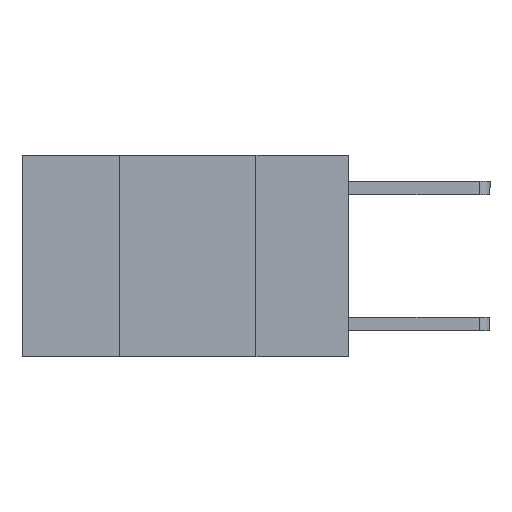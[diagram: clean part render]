
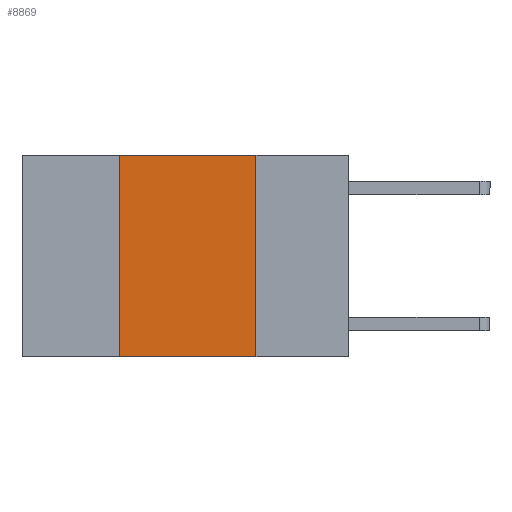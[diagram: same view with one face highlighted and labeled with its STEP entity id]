
A CAD part, left-side view. The second image highlights one B-rep face of the part: STEP entity #8869.
In plain terms, the highlighted planar face has unit normal (-1, 0, 0).
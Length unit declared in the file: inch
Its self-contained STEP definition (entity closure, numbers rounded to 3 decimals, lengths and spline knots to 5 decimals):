
#104 = EDGE_LOOP ( 'NONE', ( #6926, #2718, #4434, #5440 ) ) ;
#144 = EDGE_CURVE ( 'NONE', #7328, #1007, #1130, .T. ) ;
#227 = VECTOR ( 'NONE', #1446, 39.37008 ) ;
#294 = CARTESIAN_POINT ( 'NONE',  ( 0., 0.6, 0. ) ) ;
#667 = CARTESIAN_POINT ( 'NONE',  ( 0., 0.42, -0.37 ) ) ;
#863 = PLANE ( 'NONE',  #9332 ) ;
#979 = CARTESIAN_POINT ( 'NONE',  ( 0., 0.6, -0.37 ) ) ;
#1007 = VERTEX_POINT ( 'NONE', #3059 ) ;
#1130 = LINE ( 'NONE', #4024, #8418 ) ;
#1446 = DIRECTION ( 'NONE',  ( 0., 0., -1. ) ) ;
#1907 = LINE ( 'NONE', #4088, #3095 ) ;
#2405 = DIRECTION ( 'NONE',  ( 0., -1., 0. ) ) ;
#2706 = VECTOR ( 'NONE', #2405, 39.37008 ) ;
#2718 = ORIENTED_EDGE ( 'NONE', *, *, #5056, .F. ) ;
#3059 = CARTESIAN_POINT ( 'NONE',  ( 0., 0.42, 0. ) ) ;
#3095 = VECTOR ( 'NONE', #9239, 39.37008 ) ;
#4024 = CARTESIAN_POINT ( 'NONE',  ( 0., 0.42, 0. ) ) ;
#4088 = CARTESIAN_POINT ( 'NONE',  ( 0., 0.6, 0. ) ) ;
#4411 = VERTEX_POINT ( 'NONE', #5326 ) ;
#4434 = ORIENTED_EDGE ( 'NONE', *, *, #144, .F. ) ;
#4510 = FACE_OUTER_BOUND ( 'NONE', #104, .T. ) ;
#4603 = DIRECTION ( 'NONE',  ( 1., 0., 0. ) ) ;
#5056 = EDGE_CURVE ( 'NONE', #1007, #8896, #1907, .T. ) ;
#5326 = CARTESIAN_POINT ( 'NONE',  ( 0., 0.17, -0.37 ) ) ;
#5440 = ORIENTED_EDGE ( 'NONE', *, *, #9345, .T. ) ;
#5796 = CARTESIAN_POINT ( 'NONE',  ( 0., 0.17, 0. ) ) ;
#6628 = EDGE_CURVE ( 'NONE', #8896, #4411, #7937, .T. ) ;
#6716 = LINE ( 'NONE', #979, #2706 ) ;
#6791 = CARTESIAN_POINT ( 'NONE',  ( 0., 0.17, 0. ) ) ;
#6904 = DIRECTION ( 'NONE',  ( 0., 0., 1. ) ) ;
#6926 = ORIENTED_EDGE ( 'NONE', *, *, #6628, .F. ) ;
#7328 = VERTEX_POINT ( 'NONE', #667 ) ;
#7937 = LINE ( 'NONE', #5796, #227 ) ;
#8418 = VECTOR ( 'NONE', #6904, 39.37008 ) ;
#8757 = DIRECTION ( 'NONE',  ( 0., 0., -1. ) ) ;
#8869 = ADVANCED_FACE ( 'NONE', ( #4510 ), #863, .F. ) ;
#8896 = VERTEX_POINT ( 'NONE', #6791 ) ;
#9239 = DIRECTION ( 'NONE',  ( 0., -1., 0. ) ) ;
#9332 = AXIS2_PLACEMENT_3D ( 'NONE', #294, #4603, #8757 ) ;
#9345 = EDGE_CURVE ( 'NONE', #7328, #4411, #6716, .T. ) ;
